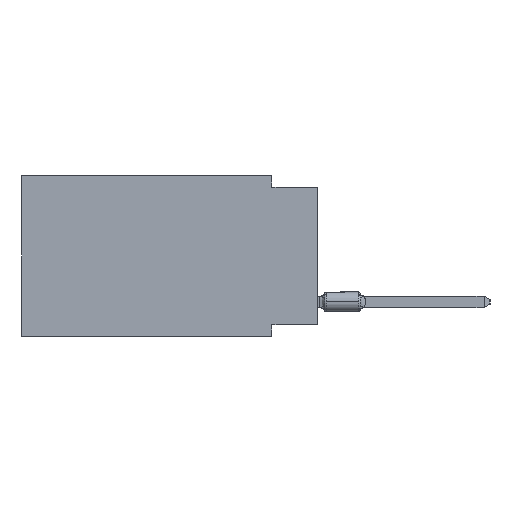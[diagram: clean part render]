
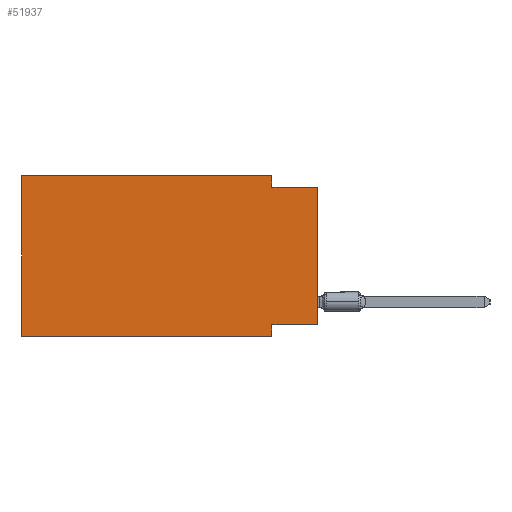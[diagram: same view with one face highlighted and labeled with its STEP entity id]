
A CAD part, left-side view. The second image highlights one B-rep face of the part: STEP entity #51937.
In plain terms, the highlighted planar face has unit normal (-1, 0, 0).
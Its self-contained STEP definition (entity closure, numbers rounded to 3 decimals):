
#329 = VECTOR ( 'NONE', #65242, 1000. ) ;
#998 = VECTOR ( 'NONE', #59638, 1000. ) ;
#1276 = EDGE_CURVE ( 'NONE', #2916, #46962, #35200, .T. ) ;
#2916 = VERTEX_POINT ( 'NONE', #28364 ) ;
#2926 = EDGE_CURVE ( 'NONE', #38847, #25481, #47705, .T. ) ;
#3358 = LINE ( 'NONE', #38060, #998 ) ;
#3500 = CARTESIAN_POINT ( 'NONE',  ( 0., 16.383, -8.89 ) ) ;
#4892 = EDGE_CURVE ( 'NONE', #27364, #25481, #53662, .T. ) ;
#4989 = DIRECTION ( 'NONE',  ( 0., 1., 0. ) ) ;
#5004 = DIRECTION ( 'NONE',  ( 0., 0., -1. ) ) ;
#5427 = EDGE_CURVE ( 'NONE', #14951, #13882, #54293, .T. ) ;
#7061 = DIRECTION ( 'NONE',  ( 0., 0., -1. ) ) ;
#9934 = CARTESIAN_POINT ( 'NONE',  ( 0., 16.383, 0. ) ) ;
#11976 = LINE ( 'NONE', #27345, #43465 ) ;
#12193 = EDGE_CURVE ( 'NONE', #38847, #60958, #37035, .T. ) ;
#13882 = VERTEX_POINT ( 'NONE', #50025 ) ;
#14017 = EDGE_CURVE ( 'NONE', #14951, #27364, #32436, .T. ) ;
#14951 = VERTEX_POINT ( 'NONE', #63580 ) ;
#15213 = EDGE_CURVE ( 'NONE', #46962, #13882, #11976, .T. ) ;
#15262 = CARTESIAN_POINT ( 'NONE',  ( 0., 2.54, -8.89 ) ) ;
#16257 = CARTESIAN_POINT ( 'NONE',  ( 0., 0., 0. ) ) ;
#17456 = DIRECTION ( 'NONE',  ( 0., -1., 0. ) ) ;
#18034 = CARTESIAN_POINT ( 'NONE',  ( 0., 2.54, -8.89 ) ) ;
#20165 = ORIENTED_EDGE ( 'NONE', *, *, #4892, .F. ) ;
#24533 = VECTOR ( 'NONE', #4989, 1000. ) ;
#25481 = VERTEX_POINT ( 'NONE', #18034 ) ;
#25762 = EDGE_CURVE ( 'NONE', #60958, #2916, #3358, .T. ) ;
#26413 = CARTESIAN_POINT ( 'NONE',  ( 0., 2.54, -0.635 ) ) ;
#27345 = CARTESIAN_POINT ( 'NONE',  ( 0., 0., -0.635 ) ) ;
#27364 = VERTEX_POINT ( 'NONE', #60962 ) ;
#28364 = CARTESIAN_POINT ( 'NONE',  ( 0., 2.54, 0. ) ) ;
#29830 = PLANE ( 'NONE',  #31326 ) ;
#30229 = VECTOR ( 'NONE', #7061, 1000. ) ;
#31326 = AXIS2_PLACEMENT_3D ( 'NONE', #69627, #57972, #46970 ) ;
#32436 = LINE ( 'NONE', #59834, #24533 ) ;
#34471 = CARTESIAN_POINT ( 'NONE',  ( 0., 2.54, 0. ) ) ;
#35200 = LINE ( 'NONE', #34471, #30229 ) ;
#37035 = LINE ( 'NONE', #65515, #64175 ) ;
#38060 = CARTESIAN_POINT ( 'NONE',  ( 0., 16.383, 0. ) ) ;
#38586 = VECTOR ( 'NONE', #47350, 1000. ) ;
#38847 = VERTEX_POINT ( 'NONE', #3500 ) ;
#42207 = FACE_OUTER_BOUND ( 'NONE', #60669, .T. ) ;
#42877 = DIRECTION ( 'NONE',  ( 0., 0., 1. ) ) ;
#43465 = VECTOR ( 'NONE', #17456, 1000. ) ;
#46499 = ORIENTED_EDGE ( 'NONE', *, *, #1276, .F. ) ;
#46962 = VERTEX_POINT ( 'NONE', #26413 ) ;
#46970 = DIRECTION ( 'NONE',  ( 0., 0., -1. ) ) ;
#47350 = DIRECTION ( 'NONE',  ( 0., -1., 0. ) ) ;
#47705 = LINE ( 'NONE', #69987, #38586 ) ;
#48318 = ORIENTED_EDGE ( 'NONE', *, *, #2926, .T. ) ;
#49716 = ORIENTED_EDGE ( 'NONE', *, *, #12193, .F. ) ;
#50025 = CARTESIAN_POINT ( 'NONE',  ( 0., 0., -0.635 ) ) ;
#50505 = ORIENTED_EDGE ( 'NONE', *, *, #14017, .F. ) ;
#51937 = ADVANCED_FACE ( 'NONE', ( #42207 ), #29830, .F. ) ;
#53662 = LINE ( 'NONE', #15262, #63326 ) ;
#54293 = LINE ( 'NONE', #16257, #329 ) ;
#56735 = ORIENTED_EDGE ( 'NONE', *, *, #15213, .F. ) ;
#57972 = DIRECTION ( 'NONE',  ( 1., 0., 0. ) ) ;
#58655 = ORIENTED_EDGE ( 'NONE', *, *, #5427, .T. ) ;
#59638 = DIRECTION ( 'NONE',  ( 0., -1., 0. ) ) ;
#59834 = CARTESIAN_POINT ( 'NONE',  ( 0., 0., -8.255 ) ) ;
#60669 = EDGE_LOOP ( 'NONE', ( #58655, #56735, #46499, #61862, #49716, #48318, #20165, #50505 ) ) ;
#60958 = VERTEX_POINT ( 'NONE', #9934 ) ;
#60962 = CARTESIAN_POINT ( 'NONE',  ( 0., 2.54, -8.255 ) ) ;
#61862 = ORIENTED_EDGE ( 'NONE', *, *, #25762, .F. ) ;
#63326 = VECTOR ( 'NONE', #5004, 1000. ) ;
#63580 = CARTESIAN_POINT ( 'NONE',  ( 0., 0., -8.255 ) ) ;
#64175 = VECTOR ( 'NONE', #42877, 1000. ) ;
#65242 = DIRECTION ( 'NONE',  ( 0., 0., 1. ) ) ;
#65515 = CARTESIAN_POINT ( 'NONE',  ( 0., 16.383, 0. ) ) ;
#69627 = CARTESIAN_POINT ( 'NONE',  ( 0., 16.383, 0. ) ) ;
#69987 = CARTESIAN_POINT ( 'NONE',  ( 0., 16.383, -8.89 ) ) ;
